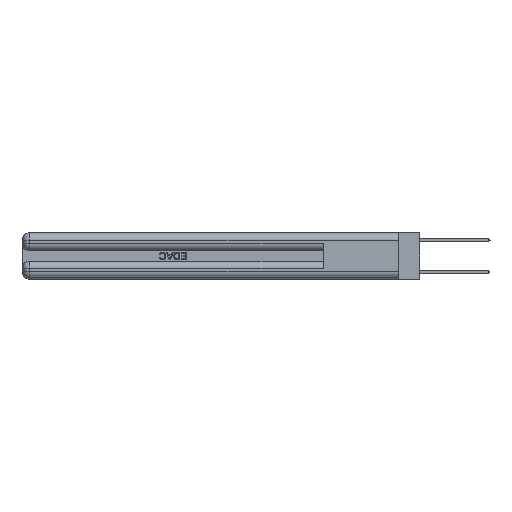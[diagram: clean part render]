
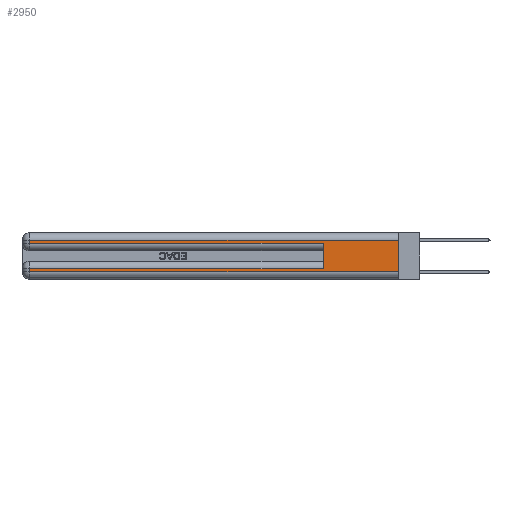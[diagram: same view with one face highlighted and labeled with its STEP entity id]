
A CAD part, left-side view. The second image highlights one B-rep face of the part: STEP entity #2950.
In plain terms, the highlighted planar face has unit normal (-1, 0, 0).
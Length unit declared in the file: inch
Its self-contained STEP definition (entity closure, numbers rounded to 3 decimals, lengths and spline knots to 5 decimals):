
#2247 = EDGE_LOOP ( 'NONE', ( #17912, #3999, #14903, #23945, #11882, #6232, #31732, #10615 ) ) ;
#2397 = VERTEX_POINT ( 'NONE', #5312 ) ;
#2950 = ADVANCED_FACE ( 'NONE', ( #5303 ), #26924, .F. ) ;
#3547 = CARTESIAN_POINT ( 'NONE',  ( 0., 2.94, 0.31 ) ) ;
#3999 = ORIENTED_EDGE ( 'NONE', *, *, #30734, .T. ) ;
#4717 = CARTESIAN_POINT ( 'NONE',  ( 0., 0., 0.37 ) ) ;
#5303 = FACE_OUTER_BOUND ( 'NONE', #2247, .T. ) ;
#5312 = CARTESIAN_POINT ( 'NONE',  ( 0., 2.94, 0.06 ) ) ;
#6208 = CARTESIAN_POINT ( 'NONE',  ( 0., 0., 0.06 ) ) ;
#6232 = ORIENTED_EDGE ( 'NONE', *, *, #14118, .T. ) ;
#6354 = VECTOR ( 'NONE', #31245, 39.37008 ) ;
#7628 = CARTESIAN_POINT ( 'NONE',  ( 0., 0., 0.37 ) ) ;
#8732 = AXIS2_PLACEMENT_3D ( 'NONE', #7628, #10418, #29688 ) ;
#8978 = LINE ( 'NONE', #34016, #6354 ) ;
#9171 = DIRECTION ( 'NONE',  ( 0., 0., -1. ) ) ;
#9294 = CARTESIAN_POINT ( 'NONE',  ( 0., 0.6, 0.085 ) ) ;
#9628 = DIRECTION ( 'NONE',  ( 0., -1., 0. ) ) ;
#10350 = DIRECTION ( 'NONE',  ( 0., 0., -1. ) ) ;
#10418 = DIRECTION ( 'NONE',  ( 1., 0., 0. ) ) ;
#10442 = EDGE_CURVE ( 'NONE', #2397, #32349, #28217, .T. ) ;
#10615 = ORIENTED_EDGE ( 'NONE', *, *, #10442, .T. ) ;
#11882 = ORIENTED_EDGE ( 'NONE', *, *, #19645, .F. ) ;
#11969 = CARTESIAN_POINT ( 'NONE',  ( 0., 2.94, 0.085 ) ) ;
#12277 = EDGE_CURVE ( 'NONE', #14090, #2397, #34529, .T. ) ;
#14090 = VERTEX_POINT ( 'NONE', #11969 ) ;
#14118 = EDGE_CURVE ( 'NONE', #27076, #14090, #8978, .T. ) ;
#14903 = ORIENTED_EDGE ( 'NONE', *, *, #27069, .T. ) ;
#16916 = CARTESIAN_POINT ( 'NONE',  ( 0., 2.94, 0.285 ) ) ;
#17030 = VERTEX_POINT ( 'NONE', #16916 ) ;
#17496 = CARTESIAN_POINT ( 'NONE',  ( 0., 2.94, 0.37 ) ) ;
#17912 = ORIENTED_EDGE ( 'NONE', *, *, #32593, .F. ) ;
#18149 = VECTOR ( 'NONE', #10350, 39.37008 ) ;
#19156 = VECTOR ( 'NONE', #35199, 39.37008 ) ;
#19645 = EDGE_CURVE ( 'NONE', #27076, #27494, #25090, .T. ) ;
#19852 = VECTOR ( 'NONE', #22952, 39.37008 ) ;
#21170 = CARTESIAN_POINT ( 'NONE',  ( 0., 0.6, 0.145 ) ) ;
#21659 = LINE ( 'NONE', #17496, #35500 ) ;
#21673 = CARTESIAN_POINT ( 'NONE',  ( 0., 0., 0.31 ) ) ;
#22952 = DIRECTION ( 'NONE',  ( 0., 0., -1. ) ) ;
#23171 = CARTESIAN_POINT ( 'NONE',  ( 0., 0., 0.31 ) ) ;
#23350 = EDGE_CURVE ( 'NONE', #17030, #27494, #29631, .T. ) ;
#23353 = CARTESIAN_POINT ( 'NONE',  ( 0., 0., 0.285 ) ) ;
#23361 = VECTOR ( 'NONE', #34260, 39.37008 ) ;
#23945 = ORIENTED_EDGE ( 'NONE', *, *, #23350, .T. ) ;
#23962 = DIRECTION ( 'NONE',  ( 0., 0., 1. ) ) ;
#24101 = CARTESIAN_POINT ( 'NONE',  ( 0., 0., 0.06 ) ) ;
#24582 = VERTEX_POINT ( 'NONE', #3547 ) ;
#25090 = LINE ( 'NONE', #21170, #31569 ) ;
#26924 = PLANE ( 'NONE',  #8732 ) ;
#27069 = EDGE_CURVE ( 'NONE', #24582, #17030, #21659, .T. ) ;
#27076 = VERTEX_POINT ( 'NONE', #9294 ) ;
#27494 = VERTEX_POINT ( 'NONE', #30347 ) ;
#27893 = VECTOR ( 'NONE', #9628, 39.37008 ) ;
#28217 = LINE ( 'NONE', #24101, #19156 ) ;
#29631 = LINE ( 'NONE', #23353, #27893 ) ;
#29688 = DIRECTION ( 'NONE',  ( 0., 0., -1. ) ) ;
#30347 = CARTESIAN_POINT ( 'NONE',  ( 0., 0.6, 0.285 ) ) ;
#30685 = LINE ( 'NONE', #23171, #23361 ) ;
#30734 = EDGE_CURVE ( 'NONE', #31043, #24582, #30685, .T. ) ;
#31043 = VERTEX_POINT ( 'NONE', #21673 ) ;
#31245 = DIRECTION ( 'NONE',  ( 0., 1., 0. ) ) ;
#31569 = VECTOR ( 'NONE', #23962, 39.37008 ) ;
#31732 = ORIENTED_EDGE ( 'NONE', *, *, #12277, .T. ) ;
#32349 = VERTEX_POINT ( 'NONE', #6208 ) ;
#32593 = EDGE_CURVE ( 'NONE', #31043, #32349, #32777, .T. ) ;
#32777 = LINE ( 'NONE', #4717, #18149 ) ;
#34016 = CARTESIAN_POINT ( 'NONE',  ( 0., 0., 0.085 ) ) ;
#34061 = CARTESIAN_POINT ( 'NONE',  ( 0., 2.94, 0.37 ) ) ;
#34260 = DIRECTION ( 'NONE',  ( 0., 1., 0. ) ) ;
#34529 = LINE ( 'NONE', #34061, #19852 ) ;
#35199 = DIRECTION ( 'NONE',  ( 0., -1., 0. ) ) ;
#35500 = VECTOR ( 'NONE', #9171, 39.37008 ) ;
